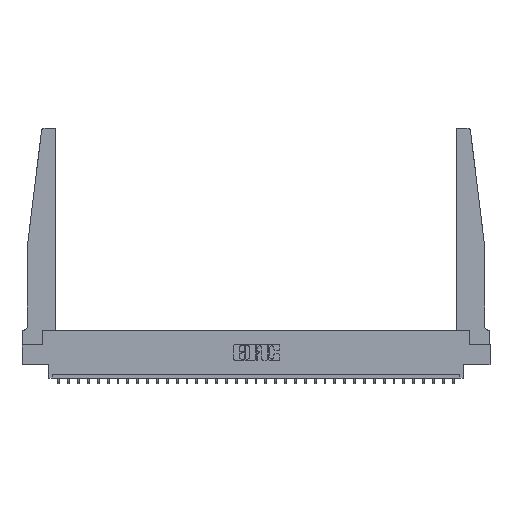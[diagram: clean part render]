
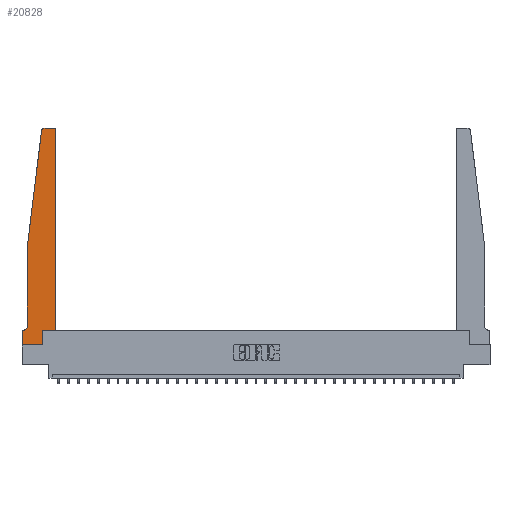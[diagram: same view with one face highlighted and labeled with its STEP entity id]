
A CAD part, top view. The second image highlights one B-rep face of the part: STEP entity #20828.
In plain terms, the highlighted planar face has unit normal (0, 0, 1).
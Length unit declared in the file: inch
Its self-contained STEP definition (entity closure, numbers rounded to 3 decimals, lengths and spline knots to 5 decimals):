
#30 = VERTEX_POINT ( 'NONE', #660 ) ;
#69 = CARTESIAN_POINT ( 'NONE',  ( 0.065, 1.25, 0.37 ) ) ;
#267 = ORIENTED_EDGE ( 'NONE', *, *, #5868, .T. ) ;
#442 = CARTESIAN_POINT ( 'NONE',  ( 0.27653, 2.72, 0.37 ) ) ;
#472 = CARTESIAN_POINT ( 'NONE',  ( 0., 0., 0.37 ) ) ;
#660 = CARTESIAN_POINT ( 'NONE',  ( 0.065, 1.25, 0.37 ) ) ;
#759 = VERTEX_POINT ( 'NONE', #25294 ) ;
#790 = VERTEX_POINT ( 'NONE', #20881 ) ;
#966 = CARTESIAN_POINT ( 'NONE',  ( 0., 0.1875, 0.37 ) ) ;
#1045 = VECTOR ( 'NONE', #27100, 39.37008 ) ;
#1070 = EDGE_CURVE ( 'NONE', #5206, #11512, #2554, .T. ) ;
#1135 = VERTEX_POINT ( 'NONE', #15551 ) ;
#1525 = CARTESIAN_POINT ( 'NONE',  ( 0.395, 2.72, 0.37 ) ) ;
#1828 = VECTOR ( 'NONE', #26465, 39.37008 ) ;
#2320 = VERTEX_POINT ( 'NONE', #17895 ) ;
#2554 = CIRCLE ( 'NONE', #22077, 0.05 ) ;
#3064 = VECTOR ( 'NONE', #20717, 39.37008 ) ;
#3269 = VECTOR ( 'NONE', #19730, 39.37008 ) ;
#3393 = CARTESIAN_POINT ( 'NONE',  ( 0., 0., 0.37 ) ) ;
#3694 = EDGE_CURVE ( 'NONE', #759, #17844, #9919, .T. ) ;
#4653 = EDGE_CURVE ( 'NONE', #2320, #790, #12986, .T. ) ;
#5165 = ORIENTED_EDGE ( 'NONE', *, *, #6748, .T. ) ;
#5206 = VERTEX_POINT ( 'NONE', #15892 ) ;
#5221 = CARTESIAN_POINT ( 'NONE',  ( 0.015, 0.1875, 0.37 ) ) ;
#5356 = FACE_OUTER_BOUND ( 'NONE', #29419, .T. ) ;
#5521 = DIRECTION ( 'NONE',  ( 0., 0., -1. ) ) ;
#5751 = ORIENTED_EDGE ( 'NONE', *, *, #12178, .T. ) ;
#5868 = EDGE_CURVE ( 'NONE', #14590, #17222, #21765, .T. ) ;
#6149 = LINE ( 'NONE', #17755, #3064 ) ;
#6610 = AXIS2_PLACEMENT_3D ( 'NONE', #1525, #8725, #28175 ) ;
#6748 = EDGE_CURVE ( 'NONE', #21037, #30, #21073, .T. ) ;
#7270 = DIRECTION ( 'NONE',  ( -0.122, -0.992, 0. ) ) ;
#8086 = EDGE_CURVE ( 'NONE', #20496, #759, #17836, .T. ) ;
#8452 = DIRECTION ( 'NONE',  ( 1., 0., 0. ) ) ;
#8725 = DIRECTION ( 'NONE',  ( 0., 0., 1. ) ) ;
#9190 = DIRECTION ( 'NONE',  ( -1., 0., 0. ) ) ;
#9262 = ORIENTED_EDGE ( 'NONE', *, *, #29282, .T. ) ;
#9604 = ORIENTED_EDGE ( 'NONE', *, *, #16890, .T. ) ;
#9919 = LINE ( 'NONE', #21996, #29781 ) ;
#10005 = CARTESIAN_POINT ( 'NONE',  ( 0.425, 0.18, 0.37 ) ) ;
#10155 = CARTESIAN_POINT ( 'NONE',  ( 0.25, 2.75, 0.37 ) ) ;
#10971 = ORIENTED_EDGE ( 'NONE', *, *, #8086, .T. ) ;
#11512 = VERTEX_POINT ( 'NONE', #5221 ) ;
#11751 = ORIENTED_EDGE ( 'NONE', *, *, #24175, .T. ) ;
#12178 = EDGE_CURVE ( 'NONE', #11512, #1135, #27862, .T. ) ;
#12354 = DIRECTION ( 'NONE',  ( 1., 0., 0. ) ) ;
#12419 = DIRECTION ( 'NONE',  ( 1., 0., 0. ) ) ;
#12547 = ORIENTED_EDGE ( 'NONE', *, *, #18350, .T. ) ;
#12733 = CARTESIAN_POINT ( 'NONE',  ( 0.425, 0.18, 0.37 ) ) ;
#12986 = LINE ( 'NONE', #10155, #1045 ) ;
#13045 = PLANE ( 'NONE',  #22050 ) ;
#13157 = ORIENTED_EDGE ( 'NONE', *, *, #3694, .T. ) ;
#14590 = VERTEX_POINT ( 'NONE', #12733 ) ;
#14926 = DIRECTION ( 'NONE',  ( 0., 0., 1. ) ) ;
#15513 = ORIENTED_EDGE ( 'NONE', *, *, #1070, .T. ) ;
#15551 = CARTESIAN_POINT ( 'NONE',  ( 0., 0.1875, 0.37 ) ) ;
#15892 = CARTESIAN_POINT ( 'NONE',  ( 0.065, 0.2375, 0.37 ) ) ;
#16890 = EDGE_CURVE ( 'NONE', #1135, #20496, #24294, .T. ) ;
#17204 = DIRECTION ( 'NONE',  ( 0., 0., 1. ) ) ;
#17222 = VERTEX_POINT ( 'NONE', #23795 ) ;
#17755 = CARTESIAN_POINT ( 'NONE',  ( 0.065, 1.25, 0.37 ) ) ;
#17836 = LINE ( 'NONE', #27410, #3269 ) ;
#17844 = VERTEX_POINT ( 'NONE', #21180 ) ;
#17895 = CARTESIAN_POINT ( 'NONE',  ( 0.395, 2.75, 0.37 ) ) ;
#18350 = EDGE_CURVE ( 'NONE', #790, #21037, #30442, .T. ) ;
#19165 = DIRECTION ( 'NONE',  ( 0., 1., 0. ) ) ;
#19730 = DIRECTION ( 'NONE',  ( 1., 0., 0. ) ) ;
#20138 = CIRCLE ( 'NONE', #6610, 0.03 ) ;
#20496 = VERTEX_POINT ( 'NONE', #3393 ) ;
#20717 = DIRECTION ( 'NONE',  ( 0., -1., 0. ) ) ;
#20828 = ADVANCED_FACE ( 'NONE', ( #5356 ), #13045, .T. ) ;
#20881 = CARTESIAN_POINT ( 'NONE',  ( 0.27653, 2.75, 0.37 ) ) ;
#21037 = VERTEX_POINT ( 'NONE', #28383 ) ;
#21073 = LINE ( 'NONE', #69, #23064 ) ;
#21180 = CARTESIAN_POINT ( 'NONE',  ( 0.2605, 0.18, 0.37 ) ) ;
#21630 = DIRECTION ( 'NONE',  ( 0., -1., 0. ) ) ;
#21765 = LINE ( 'NONE', #10005, #1828 ) ;
#21996 = CARTESIAN_POINT ( 'NONE',  ( 0.2605, 0.18, 0.37 ) ) ;
#22050 = AXIS2_PLACEMENT_3D ( 'NONE', #966, #14926, #12419 ) ;
#22077 = AXIS2_PLACEMENT_3D ( 'NONE', #22296, #5521, #26695 ) ;
#22296 = CARTESIAN_POINT ( 'NONE',  ( 0.015, 0.2375, 0.37 ) ) ;
#22439 = ORIENTED_EDGE ( 'NONE', *, *, #4653, .T. ) ;
#22468 = VECTOR ( 'NONE', #8452, 39.37008 ) ;
#23064 = VECTOR ( 'NONE', #7270, 39.37008 ) ;
#23735 = VECTOR ( 'NONE', #9190, 39.37008 ) ;
#23795 = CARTESIAN_POINT ( 'NONE',  ( 0.425, 2.72, 0.37 ) ) ;
#24175 = EDGE_CURVE ( 'NONE', #17844, #14590, #29949, .T. ) ;
#24294 = LINE ( 'NONE', #472, #27381 ) ;
#25073 = CARTESIAN_POINT ( 'NONE',  ( 0.425, 0.18, 0.37 ) ) ;
#25294 = CARTESIAN_POINT ( 'NONE',  ( 0.2605, 0., 0.37 ) ) ;
#26465 = DIRECTION ( 'NONE',  ( 0., 1., 0. ) ) ;
#26695 = DIRECTION ( 'NONE',  ( -1., 0., 0. ) ) ;
#27100 = DIRECTION ( 'NONE',  ( -1., 0., 0. ) ) ;
#27381 = VECTOR ( 'NONE', #21630, 39.37008 ) ;
#27410 = CARTESIAN_POINT ( 'NONE',  ( 0., 0., 0.37 ) ) ;
#27862 = LINE ( 'NONE', #28651, #23735 ) ;
#27912 = ORIENTED_EDGE ( 'NONE', *, *, #28243, .T. ) ;
#28175 = DIRECTION ( 'NONE',  ( 1., 0., 0. ) ) ;
#28243 = EDGE_CURVE ( 'NONE', #30, #5206, #6149, .T. ) ;
#28383 = CARTESIAN_POINT ( 'NONE',  ( 0.24675, 2.72367, 0.37 ) ) ;
#28651 = CARTESIAN_POINT ( 'NONE',  ( 0.065, 0.1875, 0.37 ) ) ;
#29282 = EDGE_CURVE ( 'NONE', #17222, #2320, #20138, .T. ) ;
#29419 = EDGE_LOOP ( 'NONE', ( #22439, #12547, #5165, #27912, #15513, #5751, #9604, #10971, #13157, #11751, #267, #9262 ) ) ;
#29781 = VECTOR ( 'NONE', #19165, 39.37008 ) ;
#29949 = LINE ( 'NONE', #25073, #22468 ) ;
#30442 = CIRCLE ( 'NONE', #30938, 0.03 ) ;
#30938 = AXIS2_PLACEMENT_3D ( 'NONE', #442, #17204, #12354 ) ;
